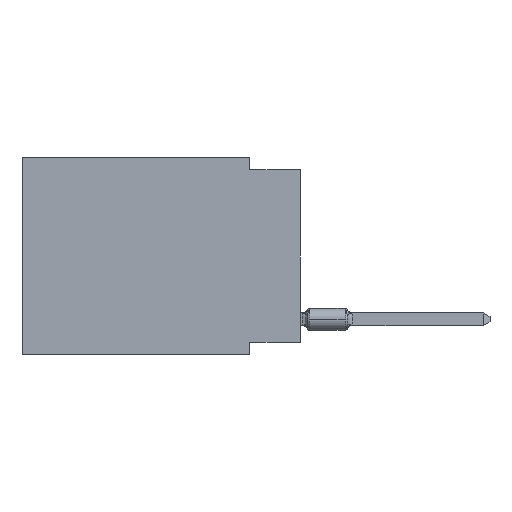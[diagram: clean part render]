
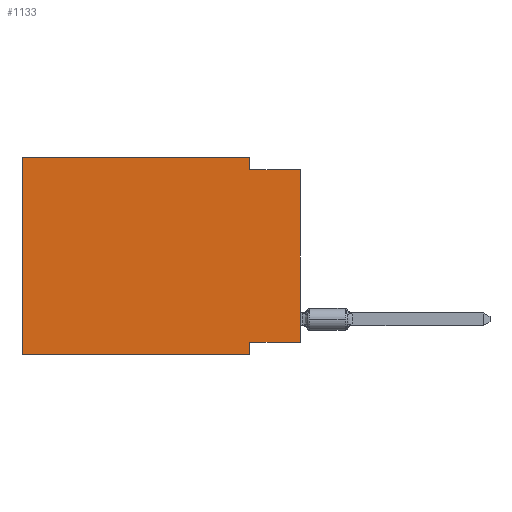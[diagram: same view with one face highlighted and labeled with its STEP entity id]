
A CAD part, left-side view. The second image highlights one B-rep face of the part: STEP entity #1133.
In plain terms, the highlighted planar face has unit normal (-1, 0, 0).
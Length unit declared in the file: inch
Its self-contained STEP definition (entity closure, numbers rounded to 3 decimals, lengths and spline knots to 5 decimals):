
#434 = EDGE_CURVE ( 'NONE', #14712, #8963, #11507, .T. ) ;
#550 = VERTEX_POINT ( 'NONE', #18066 ) ;
#880 = CARTESIAN_POINT ( 'NONE',  ( 0., 0.1, -0.39 ) ) ;
#940 = LINE ( 'NONE', #6987, #10672 ) ;
#1133 = ADVANCED_FACE ( 'NONE', ( #16843 ), #4414, .F. ) ;
#1272 = EDGE_CURVE ( 'NONE', #14712, #550, #19120, .T. ) ;
#1600 = VECTOR ( 'NONE', #13429, 39.37008 ) ;
#1624 = ORIENTED_EDGE ( 'NONE', *, *, #1272, .F. ) ;
#1757 = LINE ( 'NONE', #3436, #7167 ) ;
#1867 = VECTOR ( 'NONE', #19314, 39.37008 ) ;
#1878 = ORIENTED_EDGE ( 'NONE', *, *, #13041, .F. ) ;
#2170 = CARTESIAN_POINT ( 'NONE',  ( 0., 0.55, -0.39 ) ) ;
#2459 = CARTESIAN_POINT ( 'NONE',  ( 0., 0., -0.025 ) ) ;
#2711 = LINE ( 'NONE', #5767, #1600 ) ;
#3284 = VECTOR ( 'NONE', #11415, 39.37008 ) ;
#3436 = CARTESIAN_POINT ( 'NONE',  ( 0., 0., 0. ) ) ;
#3942 = VERTEX_POINT ( 'NONE', #17278 ) ;
#4264 = CARTESIAN_POINT ( 'NONE',  ( 0., 0.1, 0. ) ) ;
#4414 = PLANE ( 'NONE',  #9151 ) ;
#4437 = VECTOR ( 'NONE', #4993, 39.37008 ) ;
#4993 = DIRECTION ( 'NONE',  ( 0., 0., -1. ) ) ;
#5691 = ORIENTED_EDGE ( 'NONE', *, *, #6771, .F. ) ;
#5767 = CARTESIAN_POINT ( 'NONE',  ( 0., 0., -0.365 ) ) ;
#5879 = ORIENTED_EDGE ( 'NONE', *, *, #7026, .F. ) ;
#6574 = EDGE_CURVE ( 'NONE', #3942, #16087, #19327, .T. ) ;
#6771 = EDGE_CURVE ( 'NONE', #15063, #8963, #11447, .T. ) ;
#6987 = CARTESIAN_POINT ( 'NONE',  ( 0., 0.1, 0. ) ) ;
#7026 = EDGE_CURVE ( 'NONE', #16544, #15063, #2711, .T. ) ;
#7167 = VECTOR ( 'NONE', #8015, 39.37008 ) ;
#7272 = CARTESIAN_POINT ( 'NONE',  ( 0., 0.55, 0. ) ) ;
#7373 = VERTEX_POINT ( 'NONE', #4264 ) ;
#7885 = ORIENTED_EDGE ( 'NONE', *, *, #16502, .F. ) ;
#8015 = DIRECTION ( 'NONE',  ( 0., 0., 1. ) ) ;
#8963 = VERTEX_POINT ( 'NONE', #880 ) ;
#9151 = AXIS2_PLACEMENT_3D ( 'NONE', #9299, #13564, #18143 ) ;
#9299 = CARTESIAN_POINT ( 'NONE',  ( 0., 0.55, 0. ) ) ;
#9410 = ORIENTED_EDGE ( 'NONE', *, *, #6574, .F. ) ;
#9960 = CARTESIAN_POINT ( 'NONE',  ( 0., 0.1, -0.365 ) ) ;
#10672 = VECTOR ( 'NONE', #13155, 39.37008 ) ;
#11415 = DIRECTION ( 'NONE',  ( 0., -1., 0. ) ) ;
#11447 = LINE ( 'NONE', #19010, #4437 ) ;
#11507 = LINE ( 'NONE', #18972, #15469 ) ;
#13041 = EDGE_CURVE ( 'NONE', #550, #7373, #15894, .T. ) ;
#13155 = DIRECTION ( 'NONE',  ( 0., 0., -1. ) ) ;
#13429 = DIRECTION ( 'NONE',  ( 0., 1., 0. ) ) ;
#13564 = DIRECTION ( 'NONE',  ( 1., 0., 0. ) ) ;
#13839 = ORIENTED_EDGE ( 'NONE', *, *, #434, .T. ) ;
#14602 = VECTOR ( 'NONE', #17736, 39.37008 ) ;
#14712 = VERTEX_POINT ( 'NONE', #2170 ) ;
#14888 = EDGE_LOOP ( 'NONE', ( #15652, #9410, #7885, #1878, #1624, #13839, #5691, #5879 ) ) ;
#14951 = CARTESIAN_POINT ( 'NONE',  ( 0., 0., -0.025 ) ) ;
#15063 = VERTEX_POINT ( 'NONE', #9960 ) ;
#15237 = CARTESIAN_POINT ( 'NONE',  ( 0., 0., -0.365 ) ) ;
#15469 = VECTOR ( 'NONE', #15994, 39.37008 ) ;
#15652 = ORIENTED_EDGE ( 'NONE', *, *, #16382, .T. ) ;
#15894 = LINE ( 'NONE', #18882, #3284 ) ;
#15994 = DIRECTION ( 'NONE',  ( 0., -1., 0. ) ) ;
#16087 = VERTEX_POINT ( 'NONE', #2459 ) ;
#16382 = EDGE_CURVE ( 'NONE', #16544, #16087, #1757, .T. ) ;
#16502 = EDGE_CURVE ( 'NONE', #7373, #3942, #940, .T. ) ;
#16544 = VERTEX_POINT ( 'NONE', #15237 ) ;
#16843 = FACE_OUTER_BOUND ( 'NONE', #14888, .T. ) ;
#17278 = CARTESIAN_POINT ( 'NONE',  ( 0., 0.1, -0.025 ) ) ;
#17736 = DIRECTION ( 'NONE',  ( 0., -1., 0. ) ) ;
#18066 = CARTESIAN_POINT ( 'NONE',  ( 0., 0.55, 0. ) ) ;
#18143 = DIRECTION ( 'NONE',  ( 0., 0., -1. ) ) ;
#18882 = CARTESIAN_POINT ( 'NONE',  ( 0., 0.55, 0. ) ) ;
#18972 = CARTESIAN_POINT ( 'NONE',  ( 0., 0.55, -0.39 ) ) ;
#19010 = CARTESIAN_POINT ( 'NONE',  ( 0., 0.1, -0.39 ) ) ;
#19120 = LINE ( 'NONE', #7272, #1867 ) ;
#19314 = DIRECTION ( 'NONE',  ( 0., 0., 1. ) ) ;
#19327 = LINE ( 'NONE', #14951, #14602 ) ;
